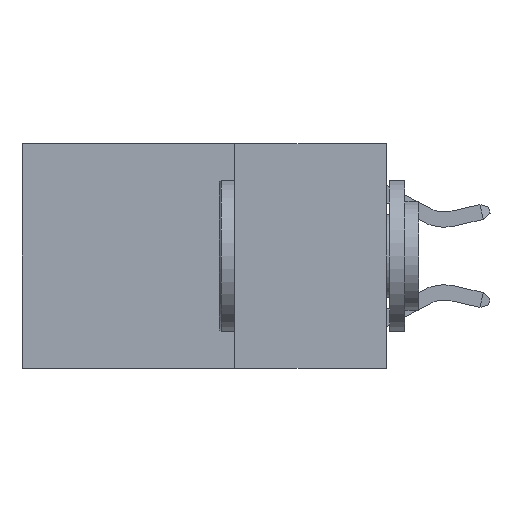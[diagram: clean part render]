
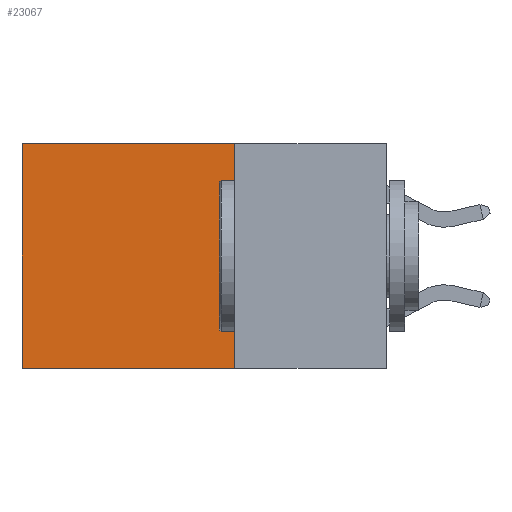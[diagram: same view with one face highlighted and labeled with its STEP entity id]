
A CAD part, left-side view. The second image highlights one B-rep face of the part: STEP entity #23067.
In plain terms, the highlighted planar face has unit normal (-1, 0, 0).
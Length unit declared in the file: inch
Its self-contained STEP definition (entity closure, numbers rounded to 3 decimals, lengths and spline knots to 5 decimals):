
#44 = LINE ( 'NONE', #3211, #617 ) ;
#316 = AXIS2_PLACEMENT_3D ( 'NONE', #12732, #14709, #7249 ) ;
#494 = EDGE_CURVE ( 'NONE', #3218, #3755, #1699, .T. ) ;
#617 = VECTOR ( 'NONE', #23495, 39.37008 ) ;
#1377 = ORIENTED_EDGE ( 'NONE', *, *, #494, .F. ) ;
#1518 = DIRECTION ( 'NONE',  ( 0., 1., 0. ) ) ;
#1699 = LINE ( 'NONE', #15632, #15448 ) ;
#1825 = FACE_OUTER_BOUND ( 'NONE', #19927, .T. ) ;
#2081 = VERTEX_POINT ( 'NONE', #9776 ) ;
#3211 = CARTESIAN_POINT ( 'NONE',  ( 0.2625, 0.25, 0. ) ) ;
#3218 = VERTEX_POINT ( 'NONE', #7284 ) ;
#3629 = PLANE ( 'NONE',  #316 ) ;
#3755 = VERTEX_POINT ( 'NONE', #23780 ) ;
#4135 = ORIENTED_EDGE ( 'NONE', *, *, #20018, .T. ) ;
#4172 = EDGE_CURVE ( 'NONE', #2081, #20933, #21544, .T. ) ;
#4772 = EDGE_CURVE ( 'NONE', #3755, #20933, #5153, .T. ) ;
#4891 = DIRECTION ( 'NONE',  ( 0., 0., -1. ) ) ;
#5153 = LINE ( 'NONE', #23725, #5739 ) ;
#5739 = VECTOR ( 'NONE', #1518, 39.37008 ) ;
#6665 = CARTESIAN_POINT ( 'NONE',  ( 0.2625, 0.6, 0. ) ) ;
#7249 = DIRECTION ( 'NONE',  ( 0., 0., -1. ) ) ;
#7284 = CARTESIAN_POINT ( 'NONE',  ( 0.2625, 0.25, 0. ) ) ;
#8926 = VECTOR ( 'NONE', #4891, 39.37008 ) ;
#9776 = CARTESIAN_POINT ( 'NONE',  ( 0.2625, 0.6, 0. ) ) ;
#12732 = CARTESIAN_POINT ( 'NONE',  ( 0.2625, 0.25, 0. ) ) ;
#14709 = DIRECTION ( 'NONE',  ( 1., 0., 0. ) ) ;
#14906 = ORIENTED_EDGE ( 'NONE', *, *, #4772, .F. ) ;
#15448 = VECTOR ( 'NONE', #21342, 39.37008 ) ;
#15632 = CARTESIAN_POINT ( 'NONE',  ( 0.2625, 0.25, 0. ) ) ;
#15826 = ORIENTED_EDGE ( 'NONE', *, *, #4172, .T. ) ;
#19927 = EDGE_LOOP ( 'NONE', ( #15826, #14906, #1377, #4135 ) ) ;
#20018 = EDGE_CURVE ( 'NONE', #3218, #2081, #44, .T. ) ;
#20933 = VERTEX_POINT ( 'NONE', #21134 ) ;
#21134 = CARTESIAN_POINT ( 'NONE',  ( 0.2625, 0.6, -0.37 ) ) ;
#21342 = DIRECTION ( 'NONE',  ( 0., 0., -1. ) ) ;
#21544 = LINE ( 'NONE', #6665, #8926 ) ;
#23067 = ADVANCED_FACE ( 'NONE', ( #1825 ), #3629, .F. ) ;
#23495 = DIRECTION ( 'NONE',  ( 0., 1., 0. ) ) ;
#23725 = CARTESIAN_POINT ( 'NONE',  ( 0.2625, 0.25, -0.37 ) ) ;
#23780 = CARTESIAN_POINT ( 'NONE',  ( 0.2625, 0.25, -0.37 ) ) ;
